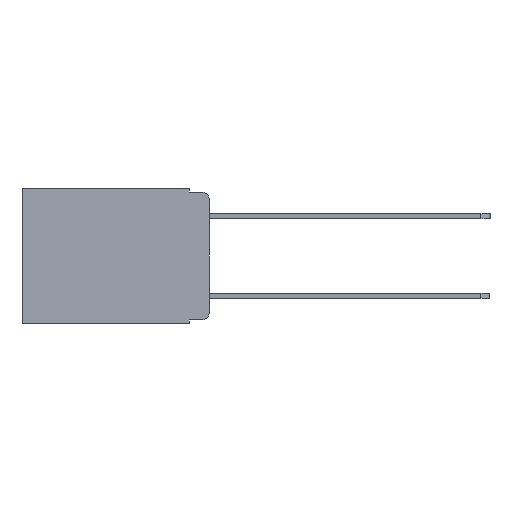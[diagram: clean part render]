
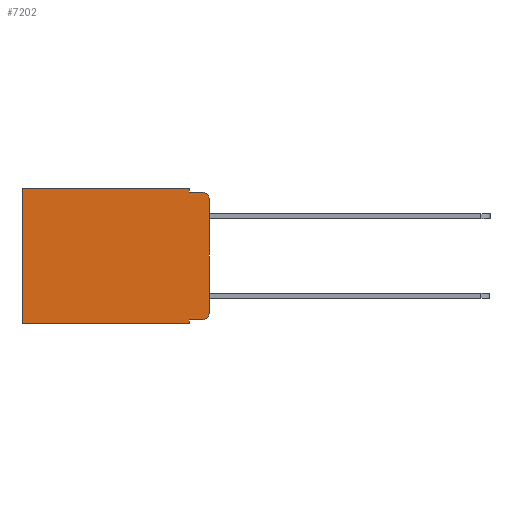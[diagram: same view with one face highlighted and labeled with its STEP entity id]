
A CAD part, left-side view. The second image highlights one B-rep face of the part: STEP entity #7202.
In plain terms, the highlighted planar face has unit normal (-1, 0, 0).
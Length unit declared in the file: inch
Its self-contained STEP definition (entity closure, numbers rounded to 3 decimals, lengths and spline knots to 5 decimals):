
#144 = EDGE_CURVE ( 'NONE', #18487, #2019, #9578, .T. ) ;
#180 = VERTEX_POINT ( 'NONE', #13368 ) ;
#298 = LINE ( 'NONE', #17215, #14912 ) ;
#573 = CARTESIAN_POINT ( 'NONE',  ( 0.298, 0.051, -0.01 ) ) ;
#1161 = DIRECTION ( 'NONE',  ( 0., 0., -1. ) ) ;
#1654 = ORIENTED_EDGE ( 'NONE', *, *, #16179, .F. ) ;
#1978 = ORIENTED_EDGE ( 'NONE', *, *, #22895, .F. ) ;
#2019 = VERTEX_POINT ( 'NONE', #14321 ) ;
#2104 = LINE ( 'NONE', #5625, #6611 ) ;
#2202 = EDGE_CURVE ( 'NONE', #4780, #15756, #10115, .T. ) ;
#2711 = LINE ( 'NONE', #23282, #22058 ) ;
#3121 = CARTESIAN_POINT ( 'NONE',  ( 0.298, 0., 0. ) ) ;
#3878 = EDGE_CURVE ( 'NONE', #15756, #23056, #8548, .T. ) ;
#4430 = CARTESIAN_POINT ( 'NONE',  ( 0.298, 0.051, 0. ) ) ;
#4440 = VECTOR ( 'NONE', #5987, 39.37008 ) ;
#4780 = VERTEX_POINT ( 'NONE', #6365 ) ;
#4889 = VERTEX_POINT ( 'NONE', #10903 ) ;
#5276 = DIRECTION ( 'NONE',  ( 0., 1., 0. ) ) ;
#5583 = ORIENTED_EDGE ( 'NONE', *, *, #3878, .T. ) ;
#5604 = LINE ( 'NONE', #17821, #15074 ) ;
#5625 = CARTESIAN_POINT ( 'NONE',  ( 0.298, 0.051, 0. ) ) ;
#5791 = CARTESIAN_POINT ( 'NONE',  ( 0.298, 0., -0.313 ) ) ;
#5987 = DIRECTION ( 'NONE',  ( 0., 1., 0. ) ) ;
#6078 = AXIS2_PLACEMENT_3D ( 'NONE', #18754, #7586, #20595 ) ;
#6365 = CARTESIAN_POINT ( 'NONE',  ( 0.298, 0.051, -0.333 ) ) ;
#6611 = VECTOR ( 'NONE', #7583, 39.37008 ) ;
#7202 = ADVANCED_FACE ( 'NONE', ( #22871 ), #17157, .F. ) ;
#7300 = VERTEX_POINT ( 'NONE', #19326 ) ;
#7583 = DIRECTION ( 'NONE',  ( 0., 0., -1. ) ) ;
#7586 = DIRECTION ( 'NONE',  ( -1., 0., 0. ) ) ;
#7659 = AXIS2_PLACEMENT_3D ( 'NONE', #13394, #13311, #13419 ) ;
#7870 = CARTESIAN_POINT ( 'NONE',  ( 0.298, 0., 0. ) ) ;
#8328 = ORIENTED_EDGE ( 'NONE', *, *, #16998, .F. ) ;
#8548 = CIRCLE ( 'NONE', #7659, 0.02 ) ;
#8625 = ORIENTED_EDGE ( 'NONE', *, *, #15402, .F. ) ;
#8786 = CARTESIAN_POINT ( 'NONE',  ( 0.298, 0., 0. ) ) ;
#9578 = LINE ( 'NONE', #8786, #4440 ) ;
#9702 = EDGE_LOOP ( 'NONE', ( #1654, #16733, #12445, #8625, #19637, #20218, #1978, #8328, #18796, #5583 ) ) ;
#9791 = DIRECTION ( 'NONE',  ( 0., 0., -1. ) ) ;
#10115 = LINE ( 'NONE', #16310, #14478 ) ;
#10480 = DIRECTION ( 'NONE',  ( 0., -1., 0. ) ) ;
#10903 = CARTESIAN_POINT ( 'NONE',  ( 0.298, 0.051, -0.343 ) ) ;
#12445 = ORIENTED_EDGE ( 'NONE', *, *, #23552, .F. ) ;
#12888 = CARTESIAN_POINT ( 'NONE',  ( 0.298, 0., -0.343 ) ) ;
#13279 = CARTESIAN_POINT ( 'NONE',  ( 0.298, 0.02, -0.333 ) ) ;
#13311 = DIRECTION ( 'NONE',  ( -1., 0., 0. ) ) ;
#13368 = CARTESIAN_POINT ( 'NONE',  ( 0.298, 0.473, -0.343 ) ) ;
#13394 = CARTESIAN_POINT ( 'NONE',  ( 0.298, 0.02, -0.313 ) ) ;
#13419 = DIRECTION ( 'NONE',  ( 0., 0., -1. ) ) ;
#13962 = LINE ( 'NONE', #3121, #15117 ) ;
#14002 = EDGE_CURVE ( 'NONE', #2019, #180, #298, .T. ) ;
#14108 = VERTEX_POINT ( 'NONE', #573 ) ;
#14321 = CARTESIAN_POINT ( 'NONE',  ( 0.298, 0.473, 0. ) ) ;
#14478 = VECTOR ( 'NONE', #10480, 39.37008 ) ;
#14912 = VECTOR ( 'NONE', #19071, 39.37008 ) ;
#15074 = VECTOR ( 'NONE', #19660, 39.37008 ) ;
#15117 = VECTOR ( 'NONE', #1161, 39.37008 ) ;
#15402 = EDGE_CURVE ( 'NONE', #18487, #14108, #2711, .T. ) ;
#15710 = EDGE_CURVE ( 'NONE', #21302, #7300, #20020, .T. ) ;
#15756 = VERTEX_POINT ( 'NONE', #13279 ) ;
#16179 = EDGE_CURVE ( 'NONE', #21302, #23056, #13962, .T. ) ;
#16310 = CARTESIAN_POINT ( 'NONE',  ( 0.298, 0.051, -0.333 ) ) ;
#16733 = ORIENTED_EDGE ( 'NONE', *, *, #15710, .T. ) ;
#16998 = EDGE_CURVE ( 'NONE', #4780, #4889, #2104, .T. ) ;
#17157 = PLANE ( 'NONE',  #21721 ) ;
#17215 = CARTESIAN_POINT ( 'NONE',  ( 0.298, 0.473, 0. ) ) ;
#17821 = CARTESIAN_POINT ( 'NONE',  ( 0.298, 0.051, -0.01 ) ) ;
#18487 = VERTEX_POINT ( 'NONE', #4430 ) ;
#18754 = CARTESIAN_POINT ( 'NONE',  ( 0.298, 0.02, -0.03 ) ) ;
#18796 = ORIENTED_EDGE ( 'NONE', *, *, #2202, .T. ) ;
#19071 = DIRECTION ( 'NONE',  ( 0., 0., -1. ) ) ;
#19128 = VECTOR ( 'NONE', #5276, 39.37008 ) ;
#19326 = CARTESIAN_POINT ( 'NONE',  ( 0.298, 0.02, -0.01 ) ) ;
#19637 = ORIENTED_EDGE ( 'NONE', *, *, #144, .T. ) ;
#19660 = DIRECTION ( 'NONE',  ( 0., -1., 0. ) ) ;
#20020 = CIRCLE ( 'NONE', #6078, 0.02 ) ;
#20218 = ORIENTED_EDGE ( 'NONE', *, *, #14002, .T. ) ;
#20595 = DIRECTION ( 'NONE',  ( 0., 0., -1. ) ) ;
#20855 = DIRECTION ( 'NONE',  ( 1., 0., 0. ) ) ;
#21155 = CARTESIAN_POINT ( 'NONE',  ( 0.298, 0., -0.03 ) ) ;
#21302 = VERTEX_POINT ( 'NONE', #21155 ) ;
#21489 = DIRECTION ( 'NONE',  ( 0., 0., -1. ) ) ;
#21721 = AXIS2_PLACEMENT_3D ( 'NONE', #7870, #20855, #9791 ) ;
#22058 = VECTOR ( 'NONE', #21489, 39.37008 ) ;
#22871 = FACE_OUTER_BOUND ( 'NONE', #9702, .T. ) ;
#22895 = EDGE_CURVE ( 'NONE', #4889, #180, #24031, .T. ) ;
#23056 = VERTEX_POINT ( 'NONE', #5791 ) ;
#23282 = CARTESIAN_POINT ( 'NONE',  ( 0.298, 0.051, 0. ) ) ;
#23552 = EDGE_CURVE ( 'NONE', #14108, #7300, #5604, .T. ) ;
#24031 = LINE ( 'NONE', #12888, #19128 ) ;
